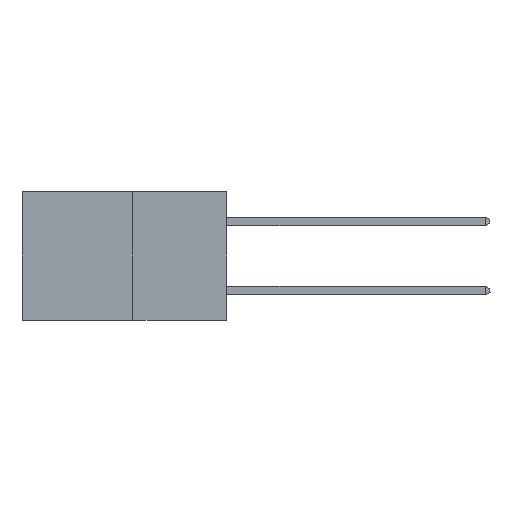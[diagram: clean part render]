
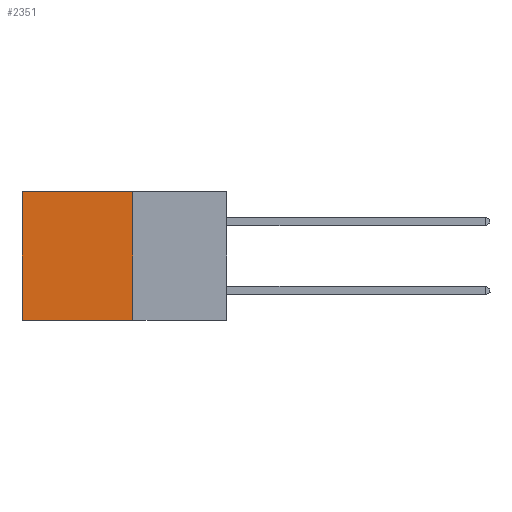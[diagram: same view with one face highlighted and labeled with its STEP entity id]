
A CAD part, left-side view. The second image highlights one B-rep face of the part: STEP entity #2351.
In plain terms, the highlighted planar face has unit normal (-1, 0, 0).
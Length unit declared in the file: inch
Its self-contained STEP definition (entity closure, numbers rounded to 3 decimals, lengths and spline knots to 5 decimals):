
#70 = CARTESIAN_POINT ( 'NONE',  ( 0.277, 0.27, 0. ) ) ;
#164 = CARTESIAN_POINT ( 'NONE',  ( 0.277, 0.27, 0. ) ) ;
#561 = DIRECTION ( 'NONE',  ( 0., 1., 0. ) ) ;
#1302 = LINE ( 'NONE', #6216, #6598 ) ;
#2042 = VERTEX_POINT ( 'NONE', #4600 ) ;
#2351 = ADVANCED_FACE ( 'NONE', ( #3646 ), #10310, .F. ) ;
#2658 = LINE ( 'NONE', #12020, #13421 ) ;
#3052 = VECTOR ( 'NONE', #12682, 39.37008 ) ;
#3646 = FACE_OUTER_BOUND ( 'NONE', #6291, .T. ) ;
#4072 = EDGE_CURVE ( 'NONE', #5580, #2042, #2658, .T. ) ;
#4105 = ORIENTED_EDGE ( 'NONE', *, *, #4072, .F. ) ;
#4600 = CARTESIAN_POINT ( 'NONE',  ( 0.277, 0.27, -0.37 ) ) ;
#5580 = VERTEX_POINT ( 'NONE', #164 ) ;
#5619 = EDGE_CURVE ( 'NONE', #9494, #9904, #11451, .T. ) ;
#6216 = CARTESIAN_POINT ( 'NONE',  ( 0.277, 0.27, -0.37 ) ) ;
#6291 = EDGE_LOOP ( 'NONE', ( #9125, #6619, #4105, #6959 ) ) ;
#6449 = EDGE_CURVE ( 'NONE', #5580, #9494, #7167, .T. ) ;
#6598 = VECTOR ( 'NONE', #13488, 39.37008 ) ;
#6619 = ORIENTED_EDGE ( 'NONE', *, *, #9538, .F. ) ;
#6838 = VECTOR ( 'NONE', #561, 39.37008 ) ;
#6959 = ORIENTED_EDGE ( 'NONE', *, *, #6449, .T. ) ;
#7167 = LINE ( 'NONE', #70, #6838 ) ;
#7831 = AXIS2_PLACEMENT_3D ( 'NONE', #10284, #10247, #10222 ) ;
#9125 = ORIENTED_EDGE ( 'NONE', *, *, #5619, .T. ) ;
#9494 = VERTEX_POINT ( 'NONE', #11436 ) ;
#9538 = EDGE_CURVE ( 'NONE', #2042, #9904, #1302, .T. ) ;
#9632 = CARTESIAN_POINT ( 'NONE',  ( 0.277, 0.59, -0.37 ) ) ;
#9904 = VERTEX_POINT ( 'NONE', #9632 ) ;
#10222 = DIRECTION ( 'NONE',  ( 0., 0., -1. ) ) ;
#10247 = DIRECTION ( 'NONE',  ( 1., 0., 0. ) ) ;
#10284 = CARTESIAN_POINT ( 'NONE',  ( 0.277, 0.27, -0.37 ) ) ;
#10310 = PLANE ( 'NONE',  #7831 ) ;
#11436 = CARTESIAN_POINT ( 'NONE',  ( 0.277, 0.59, 0. ) ) ;
#11451 = LINE ( 'NONE', #12837, #3052 ) ;
#12020 = CARTESIAN_POINT ( 'NONE',  ( 0.277, 0.27, -0.37 ) ) ;
#12081 = DIRECTION ( 'NONE',  ( 0., 0., -1. ) ) ;
#12682 = DIRECTION ( 'NONE',  ( 0., 0., -1. ) ) ;
#12837 = CARTESIAN_POINT ( 'NONE',  ( 0.277, 0.59, -0.37 ) ) ;
#13421 = VECTOR ( 'NONE', #12081, 39.37008 ) ;
#13488 = DIRECTION ( 'NONE',  ( 0., 1., 0. ) ) ;
